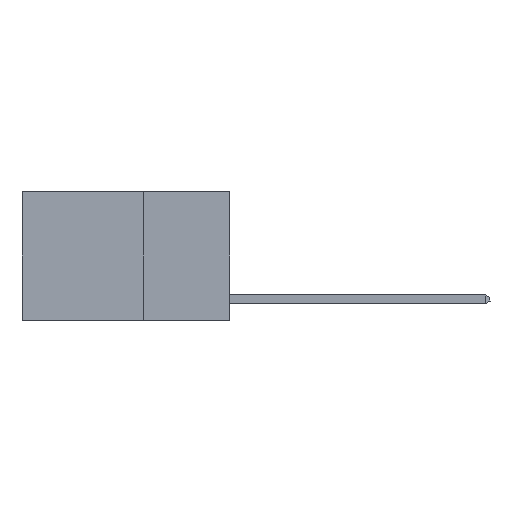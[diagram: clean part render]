
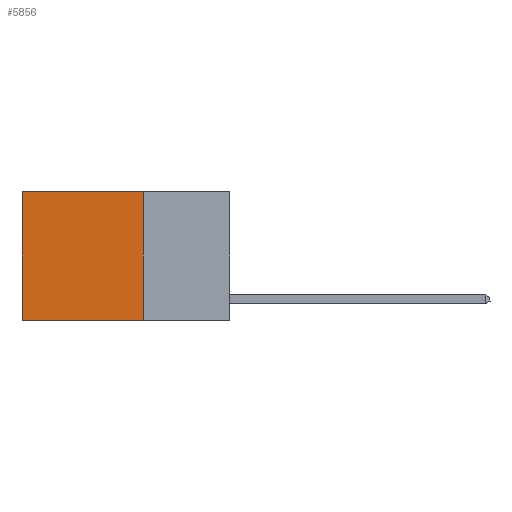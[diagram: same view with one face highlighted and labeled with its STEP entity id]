
A CAD part, left-side view. The second image highlights one B-rep face of the part: STEP entity #5856.
In plain terms, the highlighted planar face has unit normal (-1, 0, 0).
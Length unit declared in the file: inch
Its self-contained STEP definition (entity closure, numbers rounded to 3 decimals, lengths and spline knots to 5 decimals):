
#1441 = EDGE_CURVE ( 'NONE', #11809, #1821, #11245, .T. ) ;
#1549 = DIRECTION ( 'NONE',  ( 1., 0., 0. ) ) ;
#1663 = CARTESIAN_POINT ( 'NONE',  ( 0.2625, 0.25, -0.37 ) ) ;
#1786 = ORIENTED_EDGE ( 'NONE', *, *, #11141, .T. ) ;
#1821 = VERTEX_POINT ( 'NONE', #13014 ) ;
#2333 = DIRECTION ( 'NONE',  ( 0., 0., -1. ) ) ;
#2790 = LINE ( 'NONE', #4967, #10113 ) ;
#2959 = EDGE_LOOP ( 'NONE', ( #1786, #3013, #12608, #5167 ) ) ;
#3013 = ORIENTED_EDGE ( 'NONE', *, *, #5784, .F. ) ;
#3854 = DIRECTION ( 'NONE',  ( 0., 1., 0. ) ) ;
#4967 = CARTESIAN_POINT ( 'NONE',  ( 0.2625, 0.6, 0. ) ) ;
#5045 = VECTOR ( 'NONE', #2333, 39.37008 ) ;
#5167 = ORIENTED_EDGE ( 'NONE', *, *, #8944, .T. ) ;
#5784 = EDGE_CURVE ( 'NONE', #1821, #12603, #8668, .T. ) ;
#5856 = ADVANCED_FACE ( 'NONE', ( #11976 ), #9700, .F. ) ;
#5889 = VECTOR ( 'NONE', #3854, 39.37008 ) ;
#5902 = CARTESIAN_POINT ( 'NONE',  ( 0.2625, 0.25, 0. ) ) ;
#6652 = CARTESIAN_POINT ( 'NONE',  ( 0.2625, 0.25, 0. ) ) ;
#7319 = CARTESIAN_POINT ( 'NONE',  ( 0.2625, 0.6, -0.37 ) ) ;
#7553 = VERTEX_POINT ( 'NONE', #8949 ) ;
#7758 = VECTOR ( 'NONE', #9128, 39.37008 ) ;
#8668 = LINE ( 'NONE', #1663, #5889 ) ;
#8944 = EDGE_CURVE ( 'NONE', #11809, #7553, #10217, .T. ) ;
#8949 = CARTESIAN_POINT ( 'NONE',  ( 0.2625, 0.6, 0. ) ) ;
#9128 = DIRECTION ( 'NONE',  ( 0., 1., 0. ) ) ;
#9257 = CARTESIAN_POINT ( 'NONE',  ( 0.2625, 0.25, 0. ) ) ;
#9700 = PLANE ( 'NONE',  #11567 ) ;
#10113 = VECTOR ( 'NONE', #13322, 39.37008 ) ;
#10217 = LINE ( 'NONE', #5902, #7758 ) ;
#10494 = CARTESIAN_POINT ( 'NONE',  ( 0.2625, 0.25, 0. ) ) ;
#10891 = DIRECTION ( 'NONE',  ( 0., 0., -1. ) ) ;
#11141 = EDGE_CURVE ( 'NONE', #7553, #12603, #2790, .T. ) ;
#11245 = LINE ( 'NONE', #9257, #5045 ) ;
#11567 = AXIS2_PLACEMENT_3D ( 'NONE', #6652, #1549, #10891 ) ;
#11809 = VERTEX_POINT ( 'NONE', #10494 ) ;
#11976 = FACE_OUTER_BOUND ( 'NONE', #2959, .T. ) ;
#12603 = VERTEX_POINT ( 'NONE', #7319 ) ;
#12608 = ORIENTED_EDGE ( 'NONE', *, *, #1441, .F. ) ;
#13014 = CARTESIAN_POINT ( 'NONE',  ( 0.2625, 0.25, -0.37 ) ) ;
#13322 = DIRECTION ( 'NONE',  ( 0., 0., -1. ) ) ;
